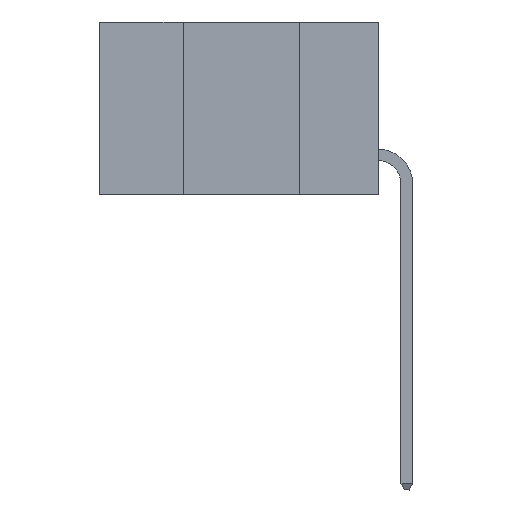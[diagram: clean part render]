
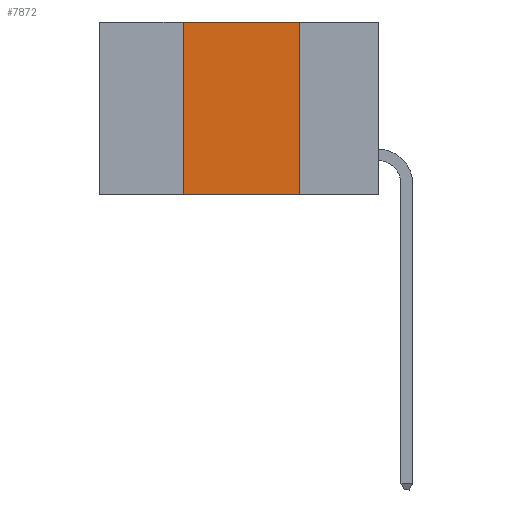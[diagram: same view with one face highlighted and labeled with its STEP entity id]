
A CAD part, left-side view. The second image highlights one B-rep face of the part: STEP entity #7872.
In plain terms, the highlighted planar face has unit normal (-1, 0, 0).
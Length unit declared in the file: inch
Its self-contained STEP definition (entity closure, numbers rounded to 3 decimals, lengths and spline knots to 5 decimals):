
#132 = ORIENTED_EDGE ( 'NONE', *, *, #5355, .T. ) ;
#214 = LINE ( 'NONE', #2530, #9084 ) ;
#242 = VERTEX_POINT ( 'NONE', #6494 ) ;
#537 = DIRECTION ( 'NONE',  ( 0., -1., 0. ) ) ;
#698 = CARTESIAN_POINT ( 'NONE',  ( 0., 0.17, -0.37 ) ) ;
#992 = EDGE_CURVE ( 'NONE', #6457, #242, #6692, .T. ) ;
#2087 = CARTESIAN_POINT ( 'NONE',  ( 0., 0.6, 0. ) ) ;
#2530 = CARTESIAN_POINT ( 'NONE',  ( 0., 0.42, -0.37 ) ) ;
#2792 = LINE ( 'NONE', #2087, #4699 ) ;
#3022 = VECTOR ( 'NONE', #7551, 39.37008 ) ;
#3058 = CARTESIAN_POINT ( 'NONE',  ( 0., 0.17, 0. ) ) ;
#3306 = VECTOR ( 'NONE', #6706, 39.37008 ) ;
#3317 = AXIS2_PLACEMENT_3D ( 'NONE', #4112, #6619, #9716 ) ;
#3566 = PLANE ( 'NONE',  #3317 ) ;
#3813 = CARTESIAN_POINT ( 'NONE',  ( 0., 0.42, 0. ) ) ;
#4077 = EDGE_CURVE ( 'NONE', #8460, #8041, #214, .T. ) ;
#4112 = CARTESIAN_POINT ( 'NONE',  ( 0., 0.6, 0. ) ) ;
#4301 = LINE ( 'NONE', #8228, #3306 ) ;
#4699 = VECTOR ( 'NONE', #537, 39.37008 ) ;
#4763 = FACE_OUTER_BOUND ( 'NONE', #6634, .T. ) ;
#4909 = DIRECTION ( 'NONE',  ( 0., 0., 1. ) ) ;
#5355 = EDGE_CURVE ( 'NONE', #8460, #242, #4301, .T. ) ;
#5844 = ORIENTED_EDGE ( 'NONE', *, *, #9531, .F. ) ;
#6457 = VERTEX_POINT ( 'NONE', #3058 ) ;
#6494 = CARTESIAN_POINT ( 'NONE',  ( 0., 0.17, -0.37 ) ) ;
#6619 = DIRECTION ( 'NONE',  ( 1., 0., 0. ) ) ;
#6634 = EDGE_LOOP ( 'NONE', ( #9847, #5844, #7322, #132 ) ) ;
#6692 = LINE ( 'NONE', #698, #3022 ) ;
#6706 = DIRECTION ( 'NONE',  ( 0., -1., 0. ) ) ;
#7322 = ORIENTED_EDGE ( 'NONE', *, *, #4077, .F. ) ;
#7551 = DIRECTION ( 'NONE',  ( 0., 0., -1. ) ) ;
#7872 = ADVANCED_FACE ( 'NONE', ( #4763 ), #3566, .F. ) ;
#8041 = VERTEX_POINT ( 'NONE', #3813 ) ;
#8228 = CARTESIAN_POINT ( 'NONE',  ( 0., 0.6, -0.37 ) ) ;
#8460 = VERTEX_POINT ( 'NONE', #9708 ) ;
#9084 = VECTOR ( 'NONE', #4909, 39.37008 ) ;
#9531 = EDGE_CURVE ( 'NONE', #8041, #6457, #2792, .T. ) ;
#9708 = CARTESIAN_POINT ( 'NONE',  ( 0., 0.42, -0.37 ) ) ;
#9716 = DIRECTION ( 'NONE',  ( 0., 0., -1. ) ) ;
#9847 = ORIENTED_EDGE ( 'NONE', *, *, #992, .F. ) ;
